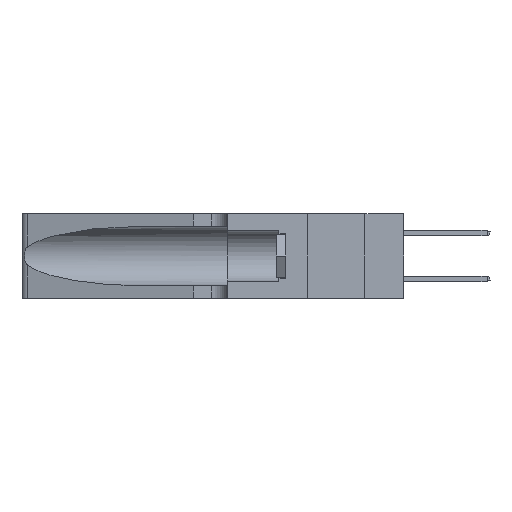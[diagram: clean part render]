
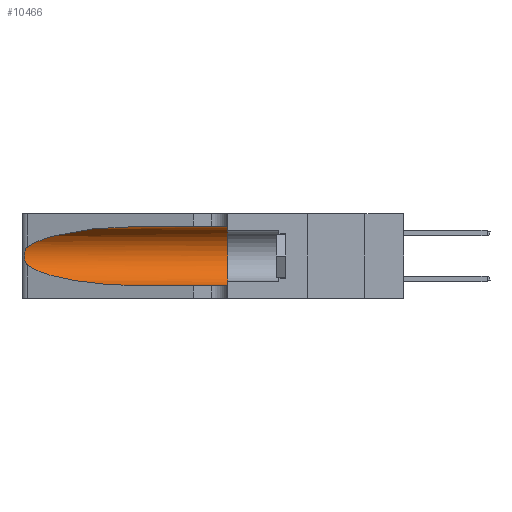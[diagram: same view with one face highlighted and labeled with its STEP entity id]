
A CAD part, left-side view. The second image highlights one B-rep face of the part: STEP entity #10466.
In plain terms, the highlighted cylindrical face has radius 3.308 mm (diameter 6.617 mm), a partial arc.
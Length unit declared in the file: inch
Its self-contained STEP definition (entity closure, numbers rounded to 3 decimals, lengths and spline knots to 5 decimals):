
#214 = VERTEX_POINT ( 'NONE', #24810 ) ;
#684 = EDGE_CURVE ( 'NONE', #214, #9036, #26401, .T. ) ;
#908 = CIRCLE ( 'NONE', #9531, 0.13025 ) ;
#1965 = AXIS2_PLACEMENT_3D ( 'NONE', #31043, #11387, #2764 ) ;
#2764 = DIRECTION ( 'NONE',  ( 0., 0., -1. ) ) ;
#2921 =( BOUNDED_CURVE ( )  B_SPLINE_CURVE ( 3, ( #32667, #15859, #27162, #10278 ),
 .UNSPECIFIED., .F., .F. ) 
 B_SPLINE_CURVE_WITH_KNOTS ( ( 4, 4 ),
 ( 1.5708, 2.84003 ),
 .UNSPECIFIED. ) 
 CURVE ( )  GEOMETRIC_REPRESENTATION_ITEM ( )  RATIONAL_B_SPLINE_CURVE ( ( 1., 0.87, 0.87, 1. ) ) 
 REPRESENTATION_ITEM ( '' )  );
#3034 = LINE ( 'NONE', #29927, #8828 ) ;
#4102 = CARTESIAN_POINT ( 'NONE',  ( 0.25787, 1.23484, 0.2124 ) ) ;
#4397 = VERTEX_POINT ( 'NONE', #7541 ) ;
#4950 = EDGE_CURVE ( 'NONE', #8933, #4397, #908, .T. ) ;
#6662 = B_SPLINE_CURVE_WITH_KNOTS ( 'NONE', 3,
 ( #32238, #23813, #21064, #4102, #23937, #6978, #26753, #9843, #29554, #12687, #32351, #15558, #35130, #18363 ),
 .UNSPECIFIED., .F., .F.,
 ( 4, 2, 2, 2, 2, 2, 4 ),
 ( 0., 0.00027, 0.00053, 0.00107, 0.0016, 0.00187, 0.00214 ),
 .UNSPECIFIED. ) ;
#6743 = ORIENTED_EDGE ( 'NONE', *, *, #10170, .T. ) ;
#6978 = CARTESIAN_POINT ( 'NONE',  ( 0.26018, 1.23835, 0.19895 ) ) ;
#7541 = CARTESIAN_POINT ( 'NONE',  ( 0.1305, 0.35, 0.05475 ) ) ;
#8312 = EDGE_CURVE ( 'NONE', #9386, #214, #6662, .T. ) ;
#8828 = VECTOR ( 'NONE', #15918, 39.37008 ) ;
#8933 = VERTEX_POINT ( 'NONE', #31835 ) ;
#9036 = VERTEX_POINT ( 'NONE', #9916 ) ;
#9386 = VERTEX_POINT ( 'NONE', #35001 ) ;
#9531 = AXIS2_PLACEMENT_3D ( 'NONE', #32266, #15462, #35038 ) ;
#9843 = CARTESIAN_POINT ( 'NONE',  ( 0.26075, 1.23896, 0.178 ) ) ;
#9916 = CARTESIAN_POINT ( 'NONE',  ( 0.1305, 0.72297, 0.05475 ) ) ;
#9995 = CYLINDRICAL_SURFACE ( 'NONE', #1965, 0.13025 ) ;
#10170 = EDGE_CURVE ( 'NONE', #26179, #9386, #2921, .T. ) ;
#10278 = CARTESIAN_POINT ( 'NONE',  ( 0.25487, 1.22718, 0.22369 ) ) ;
#10466 = ADVANCED_FACE ( 'NONE', ( #25930 ), #9995, .F. ) ;
#11387 = DIRECTION ( 'NONE',  ( 0., -1., 0. ) ) ;
#12675 = CARTESIAN_POINT ( 'NONE',  ( 0.1305, 0.72297, 0.05475 ) ) ;
#12687 = CARTESIAN_POINT ( 'NONE',  ( 0.25856, 1.23593, 0.16098 ) ) ;
#14757 = CARTESIAN_POINT ( 'NONE',  ( 0.1305, 1.61858, 0.05475 ) ) ;
#14906 = EDGE_CURVE ( 'NONE', #26179, #8933, #3034, .T. ) ;
#15462 = DIRECTION ( 'NONE',  ( 0., 1., 0. ) ) ;
#15558 = CARTESIAN_POINT ( 'NONE',  ( 0.25639, 1.23186, 0.15144 ) ) ;
#15859 = CARTESIAN_POINT ( 'NONE',  ( 0.18966, 0.96281, 0.31525 ) ) ;
#15918 = DIRECTION ( 'NONE',  ( 0., -1., 0. ) ) ;
#18363 = CARTESIAN_POINT ( 'NONE',  ( 0.25487, 1.22718, 0.14631 ) ) ;
#20488 = EDGE_CURVE ( 'NONE', #9036, #4397, #33934, .T. ) ;
#21064 = CARTESIAN_POINT ( 'NONE',  ( 0.25639, 1.23184, 0.21858 ) ) ;
#23781 = ORIENTED_EDGE ( 'NONE', *, *, #14906, .F. ) ;
#23796 = CARTESIAN_POINT ( 'NONE',  ( 0.25487, 1.22718, 0.14631 ) ) ;
#23813 = CARTESIAN_POINT ( 'NONE',  ( 0.25555, 1.22994, 0.2215 ) ) ;
#23937 = CARTESIAN_POINT ( 'NONE',  ( 0.25854, 1.2359, 0.20912 ) ) ;
#24810 = CARTESIAN_POINT ( 'NONE',  ( 0.25487, 1.22718, 0.14631 ) ) ;
#25930 = FACE_OUTER_BOUND ( 'NONE', #34481, .T. ) ;
#26179 = VERTEX_POINT ( 'NONE', #30148 ) ;
#26401 =( BOUNDED_CURVE ( )  B_SPLINE_CURVE ( 3, ( #23796, #26742, #29539, #12675 ),
 .UNSPECIFIED., .F., .F. ) 
 B_SPLINE_CURVE_WITH_KNOTS ( ( 4, 4 ),
 ( 3.44316, 4.71239 ),
 .UNSPECIFIED. ) 
 CURVE ( )  GEOMETRIC_REPRESENTATION_ITEM ( )  RATIONAL_B_SPLINE_CURVE ( ( 1., 0.87, 0.87, 1. ) ) 
 REPRESENTATION_ITEM ( '' )  );
#26534 = VECTOR ( 'NONE', #28904, 39.37008 ) ;
#26742 = CARTESIAN_POINT ( 'NONE',  ( 0.2373, 1.15595, 0.08982 ) ) ;
#26753 = CARTESIAN_POINT ( 'NONE',  ( 0.26075, 1.23896, 0.19203 ) ) ;
#27162 = CARTESIAN_POINT ( 'NONE',  ( 0.2373, 1.15595, 0.28018 ) ) ;
#27447 = ORIENTED_EDGE ( 'NONE', *, *, #4950, .F. ) ;
#28904 = DIRECTION ( 'NONE',  ( 0., -1., 0. ) ) ;
#29539 = CARTESIAN_POINT ( 'NONE',  ( 0.18966, 0.96281, 0.05475 ) ) ;
#29554 = CARTESIAN_POINT ( 'NONE',  ( 0.26017, 1.23833, 0.17102 ) ) ;
#29927 = CARTESIAN_POINT ( 'NONE',  ( 0.1305, 1.61858, 0.31525 ) ) ;
#30148 = CARTESIAN_POINT ( 'NONE',  ( 0.1305, 0.72297, 0.31525 ) ) ;
#31043 = CARTESIAN_POINT ( 'NONE',  ( 0.1305, 1.61858, 0.185 ) ) ;
#31445 = ORIENTED_EDGE ( 'NONE', *, *, #20488, .T. ) ;
#31835 = CARTESIAN_POINT ( 'NONE',  ( 0.1305, 0.35, 0.31525 ) ) ;
#32238 = CARTESIAN_POINT ( 'NONE',  ( 0.25487, 1.22718, 0.22369 ) ) ;
#32266 = CARTESIAN_POINT ( 'NONE',  ( 0.1305, 0.35, 0.185 ) ) ;
#32351 = CARTESIAN_POINT ( 'NONE',  ( 0.25789, 1.23486, 0.15765 ) ) ;
#32667 = CARTESIAN_POINT ( 'NONE',  ( 0.1305, 0.72297, 0.31525 ) ) ;
#33754 = ORIENTED_EDGE ( 'NONE', *, *, #8312, .T. ) ;
#33934 = LINE ( 'NONE', #14757, #26534 ) ;
#34481 = EDGE_LOOP ( 'NONE', ( #6743, #33754, #35357, #31445, #27447, #23781 ) ) ;
#35001 = CARTESIAN_POINT ( 'NONE',  ( 0.25487, 1.22718, 0.22369 ) ) ;
#35038 = DIRECTION ( 'NONE',  ( 0., 0., 1. ) ) ;
#35130 = CARTESIAN_POINT ( 'NONE',  ( 0.25555, 1.22993, 0.14849 ) ) ;
#35357 = ORIENTED_EDGE ( 'NONE', *, *, #684, .T. ) ;
